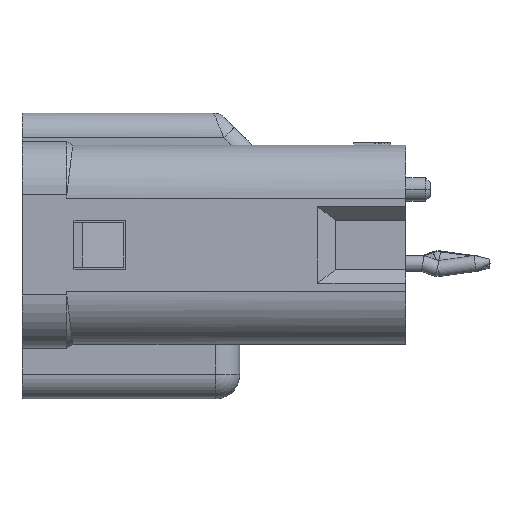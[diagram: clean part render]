
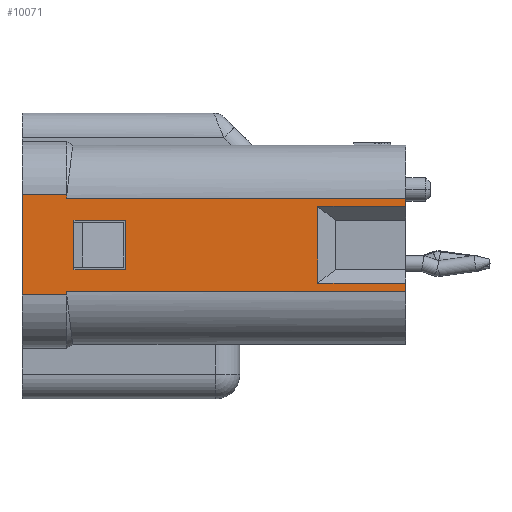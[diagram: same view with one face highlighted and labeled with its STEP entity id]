
A CAD part, left-side view. The second image highlights one B-rep face of the part: STEP entity #10071.
In plain terms, the highlighted planar face has unit normal (-1, 0, 0).
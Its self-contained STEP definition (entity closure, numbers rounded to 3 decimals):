
#209 = CARTESIAN_POINT ( 'NONE',  ( 0., 7.225, -16.804 ) ) ;
#272 = VERTEX_POINT ( 'NONE', #19960 ) ;
#798 = CARTESIAN_POINT ( 'NONE',  ( 0., 4.35, -17.104 ) ) ;
#808 = VECTOR ( 'NONE', #5189, 1000. ) ;
#1090 = CARTESIAN_POINT ( 'NONE',  ( 0., 8.1, -3.404 ) ) ;
#1151 = LINE ( 'NONE', #21803, #24611 ) ;
#1193 = CARTESIAN_POINT ( 'NONE',  ( 0., 8.1, -3.404 ) ) ;
#1375 = VECTOR ( 'NONE', #15617, 1000. ) ;
#1432 = ORIENTED_EDGE ( 'NONE', *, *, #22899, .T. ) ;
#1549 = VECTOR ( 'NONE', #8527, 1000. ) ;
#2001 = CARTESIAN_POINT ( 'NONE',  ( 0., 8.25, -17.104 ) ) ;
#2049 = LINE ( 'NONE', #10017, #10919 ) ;
#2152 = DIRECTION ( 'NONE',  ( 0., 0., 1. ) ) ;
#2524 = VERTEX_POINT ( 'NONE', #3931 ) ;
#2725 = VERTEX_POINT ( 'NONE', #19859 ) ;
#2969 = CARTESIAN_POINT ( 'NONE',  ( 0., 7.225, -14.704 ) ) ;
#3065 = VERTEX_POINT ( 'NONE', #21696 ) ;
#3095 = VECTOR ( 'NONE', #7946, 1000. ) ;
#3112 = VECTOR ( 'NONE', #4439, 1000. ) ;
#3681 = VERTEX_POINT ( 'NONE', #3961 ) ;
#3764 = LINE ( 'NONE', #20930, #15211 ) ;
#3931 = CARTESIAN_POINT ( 'NONE',  ( 0., 4.2, -17.104 ) ) ;
#3961 = CARTESIAN_POINT ( 'NONE',  ( 0., 8.1, -3.404 ) ) ;
#4242 = ORIENTED_EDGE ( 'NONE', *, *, #7948, .F. ) ;
#4330 = VERTEX_POINT ( 'NONE', #12498 ) ;
#4425 = VERTEX_POINT ( 'NONE', #20666 ) ;
#4439 = DIRECTION ( 'NONE',  ( 0., -1., 0. ) ) ;
#4452 = CARTESIAN_POINT ( 'NONE',  ( 0., 4.675, -6.954 ) ) ;
#4669 = DIRECTION ( 'NONE',  ( 0., 0., -1. ) ) ;
#4917 = ORIENTED_EDGE ( 'NONE', *, *, #10210, .T. ) ;
#5189 = DIRECTION ( 'NONE',  ( 0., -1., 0. ) ) ;
#5219 = CARTESIAN_POINT ( 'NONE',  ( 0., 8.25, -18.904 ) ) ;
#5609 = DIRECTION ( 'NONE',  ( 0., 0., -1. ) ) ;
#5612 = VECTOR ( 'NONE', #4669, 1000. ) ;
#5629 = VECTOR ( 'NONE', #10148, 1000. ) ;
#5867 = EDGE_CURVE ( 'NONE', #24070, #4330, #22789, .T. ) ;
#5999 = EDGE_LOOP ( 'NONE', ( #21698, #24296, #22196, #11374 ) ) ;
#6122 = CARTESIAN_POINT ( 'NONE',  ( 0., 7.225, -16.804 ) ) ;
#6305 = LINE ( 'NONE', #2969, #3112 ) ;
#6373 = LINE ( 'NONE', #23302, #18019 ) ;
#6377 = CARTESIAN_POINT ( 'NONE',  ( 0., 4.35, -3.404 ) ) ;
#6426 = EDGE_CURVE ( 'NONE', #13612, #16735, #6305, .T. ) ;
#6463 = ORIENTED_EDGE ( 'NONE', *, *, #13362, .F. ) ;
#6527 = VERTEX_POINT ( 'NONE', #22487 ) ;
#6551 = LINE ( 'NONE', #1193, #5612 ) ;
#6773 = EDGE_CURVE ( 'NONE', #19477, #13612, #15150, .T. ) ;
#6890 = CARTESIAN_POINT ( 'NONE',  ( 0., 4.675, -3.404 ) ) ;
#7098 = VECTOR ( 'NONE', #22144, 1000. ) ;
#7412 = EDGE_CURVE ( 'NONE', #15105, #24070, #22511, .T. ) ;
#7424 = PLANE ( 'NONE',  #17163 ) ;
#7606 = CARTESIAN_POINT ( 'NONE',  ( 0., 7.775, -6.954 ) ) ;
#7946 = DIRECTION ( 'NONE',  ( 0., 1., 0. ) ) ;
#7948 = EDGE_CURVE ( 'NONE', #2725, #2524, #23700, .T. ) ;
#8527 = DIRECTION ( 'NONE',  ( 0., -1., 0. ) ) ;
#8701 = CARTESIAN_POINT ( 'NONE',  ( 0., 8.25, -17.104 ) ) ;
#8940 = LINE ( 'NONE', #1090, #808 ) ;
#9367 = LINE ( 'NONE', #16965, #20041 ) ;
#9419 = DIRECTION ( 'NONE',  ( 0., 0., 1. ) ) ;
#9499 = ORIENTED_EDGE ( 'NONE', *, *, #7412, .F. ) ;
#9686 = EDGE_CURVE ( 'NONE', #3065, #4425, #9829, .T. ) ;
#9829 = LINE ( 'NONE', #4452, #3095 ) ;
#10017 = CARTESIAN_POINT ( 'NONE',  ( 0., 4.35, -17.104 ) ) ;
#10071 = ADVANCED_FACE ( 'NONE', ( #20394, #11188 ), #7424, .T. ) ;
#10148 = DIRECTION ( 'NONE',  ( 0., 0., -1. ) ) ;
#10210 = EDGE_CURVE ( 'NONE', #3681, #4330, #6551, .T. ) ;
#10596 = ORIENTED_EDGE ( 'NONE', *, *, #18100, .T. ) ;
#10706 = EDGE_CURVE ( 'NONE', #15440, #3065, #18117, .T. ) ;
#10919 = VECTOR ( 'NONE', #15126, 1000. ) ;
#10961 = EDGE_CURVE ( 'NONE', #272, #2524, #3764, .T. ) ;
#11188 = FACE_OUTER_BOUND ( 'NONE', #11808, .T. ) ;
#11374 = ORIENTED_EDGE ( 'NONE', *, *, #6773, .T. ) ;
#11808 = EDGE_LOOP ( 'NONE', ( #10596, #6463, #4917, #18135, #9499, #15361, #23236, #4242, #1432, #12830, #19903, #16470 ) ) ;
#12243 = CARTESIAN_POINT ( 'NONE',  ( 0., 7.775, -3.404 ) ) ;
#12498 = CARTESIAN_POINT ( 'NONE',  ( 0., 8.1, -17.104 ) ) ;
#12830 = ORIENTED_EDGE ( 'NONE', *, *, #12897, .F. ) ;
#12897 = EDGE_CURVE ( 'NONE', #15440, #21828, #1151, .T. ) ;
#12942 = VERTEX_POINT ( 'NONE', #12243 ) ;
#13175 = DIRECTION ( 'NONE',  ( -1., 0., 0. ) ) ;
#13362 = EDGE_CURVE ( 'NONE', #3681, #12942, #8940, .T. ) ;
#13612 = VERTEX_POINT ( 'NONE', #14029 ) ;
#14029 = CARTESIAN_POINT ( 'NONE',  ( 0., 7.225, -14.704 ) ) ;
#15041 = CARTESIAN_POINT ( 'NONE',  ( 0., 8.1, -18.904 ) ) ;
#15105 = VERTEX_POINT ( 'NONE', #16553 ) ;
#15126 = DIRECTION ( 'NONE',  ( 0., 0., 1. ) ) ;
#15150 = LINE ( 'NONE', #209, #16247 ) ;
#15211 = VECTOR ( 'NONE', #2152, 1000. ) ;
#15361 = ORIENTED_EDGE ( 'NONE', *, *, #16578, .F. ) ;
#15440 = VERTEX_POINT ( 'NONE', #6890 ) ;
#15617 = DIRECTION ( 'NONE',  ( 0., 1., 0. ) ) ;
#16230 = DIRECTION ( 'NONE',  ( 0., -1., 0. ) ) ;
#16247 = VECTOR ( 'NONE', #9419, 1000. ) ;
#16433 = VECTOR ( 'NONE', #24414, 1000. ) ;
#16470 = ORIENTED_EDGE ( 'NONE', *, *, #9686, .T. ) ;
#16553 = CARTESIAN_POINT ( 'NONE',  ( 0., 8.25, -18.904 ) ) ;
#16578 = EDGE_CURVE ( 'NONE', #272, #15105, #21200, .T. ) ;
#16735 = VERTEX_POINT ( 'NONE', #18345 ) ;
#16854 = LINE ( 'NONE', #7606, #16433 ) ;
#16961 = EDGE_CURVE ( 'NONE', #16735, #6527, #9367, .T. ) ;
#16965 = CARTESIAN_POINT ( 'NONE',  ( 0., 5.225, -14.704 ) ) ;
#17163 = AXIS2_PLACEMENT_3D ( 'NONE', #15041, #13175, #20752 ) ;
#17202 = DIRECTION ( 'NONE',  ( 0., -1., 0. ) ) ;
#17482 = CARTESIAN_POINT ( 'NONE',  ( 0., 4.2, -18.904 ) ) ;
#18019 = VECTOR ( 'NONE', #21684, 1000. ) ;
#18100 = EDGE_CURVE ( 'NONE', #4425, #12942, #16854, .T. ) ;
#18117 = LINE ( 'NONE', #19709, #5629 ) ;
#18135 = ORIENTED_EDGE ( 'NONE', *, *, #5867, .F. ) ;
#18345 = CARTESIAN_POINT ( 'NONE',  ( 0., 5.225, -14.704 ) ) ;
#19477 = VERTEX_POINT ( 'NONE', #6122 ) ;
#19709 = CARTESIAN_POINT ( 'NONE',  ( 0., 4.675, -3.404 ) ) ;
#19859 = CARTESIAN_POINT ( 'NONE',  ( 0., 4.35, -17.104 ) ) ;
#19903 = ORIENTED_EDGE ( 'NONE', *, *, #10706, .T. ) ;
#19960 = CARTESIAN_POINT ( 'NONE',  ( 0., 4.2, -18.904 ) ) ;
#20041 = VECTOR ( 'NONE', #5609, 1000. ) ;
#20394 = FACE_BOUND ( 'NONE', #5999, .T. ) ;
#20519 = EDGE_CURVE ( 'NONE', #6527, #19477, #6373, .T. ) ;
#20666 = CARTESIAN_POINT ( 'NONE',  ( 0., 7.775, -6.954 ) ) ;
#20752 = DIRECTION ( 'NONE',  ( 0., -1., 0. ) ) ;
#20930 = CARTESIAN_POINT ( 'NONE',  ( 0., 4.2, -18.904 ) ) ;
#21200 = LINE ( 'NONE', #17482, #1375 ) ;
#21684 = DIRECTION ( 'NONE',  ( 0., 1., 0. ) ) ;
#21696 = CARTESIAN_POINT ( 'NONE',  ( 0., 4.675, -6.954 ) ) ;
#21698 = ORIENTED_EDGE ( 'NONE', *, *, #6426, .T. ) ;
#21803 = CARTESIAN_POINT ( 'NONE',  ( 0., 4.675, -3.404 ) ) ;
#21828 = VERTEX_POINT ( 'NONE', #6377 ) ;
#22144 = DIRECTION ( 'NONE',  ( 0., 0., 1. ) ) ;
#22196 = ORIENTED_EDGE ( 'NONE', *, *, #20519, .T. ) ;
#22487 = CARTESIAN_POINT ( 'NONE',  ( 0., 5.225, -16.804 ) ) ;
#22511 = LINE ( 'NONE', #5219, #7098 ) ;
#22789 = LINE ( 'NONE', #2001, #23729 ) ;
#22899 = EDGE_CURVE ( 'NONE', #2725, #21828, #2049, .T. ) ;
#23236 = ORIENTED_EDGE ( 'NONE', *, *, #10961, .T. ) ;
#23302 = CARTESIAN_POINT ( 'NONE',  ( 0., 5.225, -16.804 ) ) ;
#23700 = LINE ( 'NONE', #798, #1549 ) ;
#23729 = VECTOR ( 'NONE', #17202, 1000. ) ;
#24070 = VERTEX_POINT ( 'NONE', #8701 ) ;
#24296 = ORIENTED_EDGE ( 'NONE', *, *, #16961, .T. ) ;
#24414 = DIRECTION ( 'NONE',  ( 0., 0., 1. ) ) ;
#24611 = VECTOR ( 'NONE', #16230, 1000. ) ;
